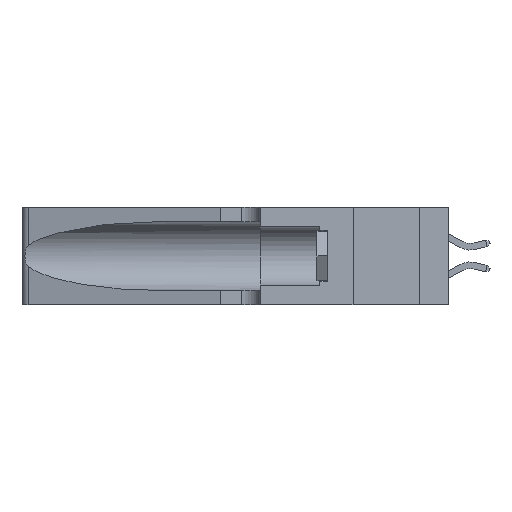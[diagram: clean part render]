
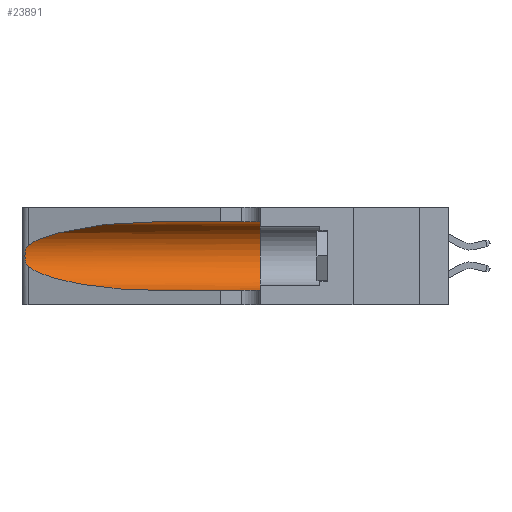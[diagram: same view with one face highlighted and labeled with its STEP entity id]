
A CAD part, left-side view. The second image highlights one B-rep face of the part: STEP entity #23891.
In plain terms, the highlighted cylindrical face has radius 3.308 mm (diameter 6.617 mm), a partial arc.
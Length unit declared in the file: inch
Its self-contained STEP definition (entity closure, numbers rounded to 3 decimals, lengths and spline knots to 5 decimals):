
#761 = CARTESIAN_POINT ( 'NONE',  ( 0.25787, 1.23484, 0.2124 ) ) ;
#1767 = CARTESIAN_POINT ( 'NONE',  ( 0.1305, 1.61858, 0.185 ) ) ;
#3407 = CARTESIAN_POINT ( 'NONE',  ( 0.1305, 0.72297, 0.31525 ) ) ;
#3910 = CARTESIAN_POINT ( 'NONE',  ( 0.26018, 1.23835, 0.19895 ) ) ;
#4897 = DIRECTION ( 'NONE',  ( 0., 0., -1. ) ) ;
#5921 = CARTESIAN_POINT ( 'NONE',  ( 0.1305, 1.61858, 0.31525 ) ) ;
#5979 = CARTESIAN_POINT ( 'NONE',  ( 0.25487, 1.22718, 0.22369 ) ) ;
#6265 = CARTESIAN_POINT ( 'NONE',  ( 0.1305, 0.35, 0.31525 ) ) ;
#6461 = EDGE_LOOP ( 'NONE', ( #32056, #34267, #28553, #6544, #28154, #11522 ) ) ;
#6544 = ORIENTED_EDGE ( 'NONE', *, *, #15848, .T. ) ;
#6564 = CARTESIAN_POINT ( 'NONE',  ( 0.1305, 0.35, 0.05475 ) ) ;
#6980 = CARTESIAN_POINT ( 'NONE',  ( 0.26075, 1.23896, 0.178 ) ) ;
#7139 = EDGE_CURVE ( 'NONE', #33287, #38608, #38921, .T. ) ;
#8838 = LINE ( 'NONE', #5921, #22999 ) ;
#8965 = CARTESIAN_POINT ( 'NONE',  ( 0.1305, 0.72297, 0.31525 ) ) ;
#9853 = CARTESIAN_POINT ( 'NONE',  ( 0.1305, 0.72297, 0.05475 ) ) ;
#10076 = CARTESIAN_POINT ( 'NONE',  ( 0.25856, 1.23593, 0.16098 ) ) ;
#10826 = DIRECTION ( 'NONE',  ( 0., -1., 0. ) ) ;
#11374 = CARTESIAN_POINT ( 'NONE',  ( 0.1305, 0.35, 0.185 ) ) ;
#11522 = ORIENTED_EDGE ( 'NONE', *, *, #13144, .F. ) ;
#12964 = CARTESIAN_POINT ( 'NONE',  ( 0.25487, 1.22718, 0.22369 ) ) ;
#13093 = CARTESIAN_POINT ( 'NONE',  ( 0.25639, 1.23186, 0.15144 ) ) ;
#13144 = EDGE_CURVE ( 'NONE', #35494, #13855, #8838, .T. ) ;
#13850 = CARTESIAN_POINT ( 'NONE',  ( 0.1305, 1.61858, 0.05475 ) ) ;
#13855 = VERTEX_POINT ( 'NONE', #6265 ) ;
#14396 = DIRECTION ( 'NONE',  ( 0., 0., 1. ) ) ;
#14922 = LINE ( 'NONE', #13850, #37226 ) ;
#15177 = DIRECTION ( 'NONE',  ( 0., -1., 0. ) ) ;
#15848 = EDGE_CURVE ( 'NONE', #38608, #27887, #14922, .T. ) ;
#15923 = FACE_OUTER_BOUND ( 'NONE', #6461, .T. ) ;
#15973 = CARTESIAN_POINT ( 'NONE',  ( 0.25555, 1.22994, 0.2215 ) ) ;
#16112 = CARTESIAN_POINT ( 'NONE',  ( 0.25487, 1.22718, 0.14631 ) ) ;
#18829 = CARTESIAN_POINT ( 'NONE',  ( 0.18966, 0.96281, 0.05475 ) ) ;
#19031 = CARTESIAN_POINT ( 'NONE',  ( 0.25639, 1.23184, 0.21858 ) ) ;
#21586 = CARTESIAN_POINT ( 'NONE',  ( 0.18966, 0.96281, 0.31525 ) ) ;
#21866 = CARTESIAN_POINT ( 'NONE',  ( 0.1305, 0.72297, 0.05475 ) ) ;
#21881 = CARTESIAN_POINT ( 'NONE',  ( 0.2373, 1.15595, 0.08982 ) ) ;
#22091 = CARTESIAN_POINT ( 'NONE',  ( 0.25854, 1.2359, 0.20912 ) ) ;
#22999 = VECTOR ( 'NONE', #15177, 39.37008 ) ;
#23012 = CYLINDRICAL_SURFACE ( 'NONE', #27734, 0.13025 ) ;
#23040 = DIRECTION ( 'NONE',  ( 0., -1., 0. ) ) ;
#23891 = ADVANCED_FACE ( 'NONE', ( #15923 ), #23012, .F. ) ;
#24197 = EDGE_CURVE ( 'NONE', #35494, #28972, #36151, .T. ) ;
#24607 = CARTESIAN_POINT ( 'NONE',  ( 0.25487, 1.22718, 0.22369 ) ) ;
#25110 = CARTESIAN_POINT ( 'NONE',  ( 0.26075, 1.23896, 0.19203 ) ) ;
#25285 = CIRCLE ( 'NONE', #29807, 0.13025 ) ;
#27734 = AXIS2_PLACEMENT_3D ( 'NONE', #1767, #23040, #4897 ) ;
#27887 = VERTEX_POINT ( 'NONE', #6564 ) ;
#27955 = CARTESIAN_POINT ( 'NONE',  ( 0.25487, 1.22718, 0.14631 ) ) ;
#28154 = ORIENTED_EDGE ( 'NONE', *, *, #38948, .F. ) ;
#28166 = CARTESIAN_POINT ( 'NONE',  ( 0.26017, 1.23833, 0.17102 ) ) ;
#28553 = ORIENTED_EDGE ( 'NONE', *, *, #7139, .T. ) ;
#28972 = VERTEX_POINT ( 'NONE', #5979 ) ;
#29268 = B_SPLINE_CURVE_WITH_KNOTS ( 'NONE', 3,
 ( #12964, #15973, #19031, #761, #22091, #3910, #25110, #6980, #28166, #10076, #31227, #13093, #34273, #16112 ),
 .UNSPECIFIED., .F., .F.,
 ( 4, 2, 2, 2, 2, 2, 4 ),
 ( 0., 0.00027, 0.00053, 0.00107, 0.0016, 0.00187, 0.00214 ),
 .UNSPECIFIED. ) ;
#29807 = AXIS2_PLACEMENT_3D ( 'NONE', #11374, #32541, #14396 ) ;
#31227 = CARTESIAN_POINT ( 'NONE',  ( 0.25789, 1.23486, 0.15765 ) ) ;
#32056 = ORIENTED_EDGE ( 'NONE', *, *, #24197, .T. ) ;
#32247 = CARTESIAN_POINT ( 'NONE',  ( 0.25487, 1.22718, 0.14631 ) ) ;
#32541 = DIRECTION ( 'NONE',  ( 0., 1., 0. ) ) ;
#33287 = VERTEX_POINT ( 'NONE', #32247 ) ;
#34267 = ORIENTED_EDGE ( 'NONE', *, *, #35579, .T. ) ;
#34273 = CARTESIAN_POINT ( 'NONE',  ( 0.25555, 1.22993, 0.14849 ) ) ;
#35494 = VERTEX_POINT ( 'NONE', #8965 ) ;
#35579 = EDGE_CURVE ( 'NONE', #28972, #33287, #29268, .T. ) ;
#36151 =( BOUNDED_CURVE ( )  B_SPLINE_CURVE ( 3, ( #3407, #21586, #36692, #24607 ),
 .UNSPECIFIED., .F., .F. ) 
 B_SPLINE_CURVE_WITH_KNOTS ( ( 4, 4 ),
 ( 1.5708, 2.84003 ),
 .UNSPECIFIED. ) 
 CURVE ( )  GEOMETRIC_REPRESENTATION_ITEM ( )  RATIONAL_B_SPLINE_CURVE ( ( 1., 0.87, 0.87, 1. ) ) 
 REPRESENTATION_ITEM ( '' )  );
#36692 = CARTESIAN_POINT ( 'NONE',  ( 0.2373, 1.15595, 0.28018 ) ) ;
#37226 = VECTOR ( 'NONE', #10826, 39.37008 ) ;
#38608 = VERTEX_POINT ( 'NONE', #21866 ) ;
#38921 =( BOUNDED_CURVE ( )  B_SPLINE_CURVE ( 3, ( #27955, #21881, #18829, #9853 ),
 .UNSPECIFIED., .F., .F. ) 
 B_SPLINE_CURVE_WITH_KNOTS ( ( 4, 4 ),
 ( 3.44316, 4.71239 ),
 .UNSPECIFIED. ) 
 CURVE ( )  GEOMETRIC_REPRESENTATION_ITEM ( )  RATIONAL_B_SPLINE_CURVE ( ( 1., 0.87, 0.87, 1. ) ) 
 REPRESENTATION_ITEM ( '' )  );
#38948 = EDGE_CURVE ( 'NONE', #13855, #27887, #25285, .T. ) ;
